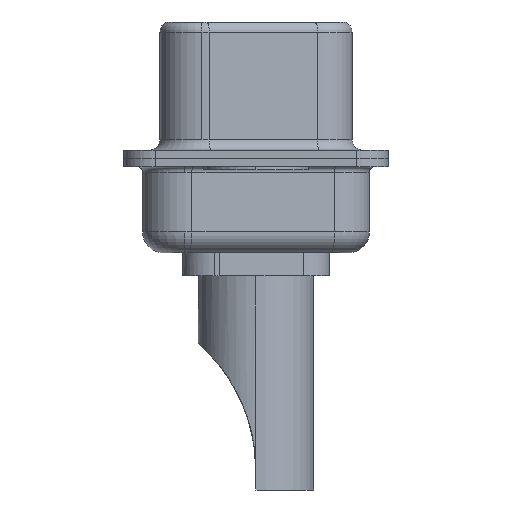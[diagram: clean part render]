
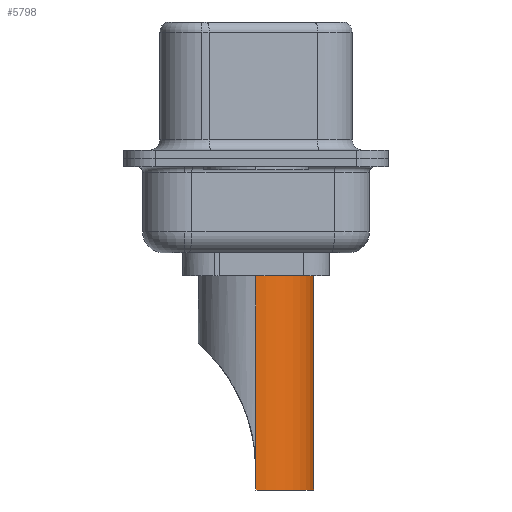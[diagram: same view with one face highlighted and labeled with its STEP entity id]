
A CAD part, left-side view. The second image highlights one B-rep face of the part: STEP entity #5798.
In plain terms, the highlighted cylindrical face has radius 2.75 mm (diameter 5.5 mm), a partial arc.
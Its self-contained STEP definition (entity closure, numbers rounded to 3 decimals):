
#401 = EDGE_CURVE ( 'NONE', #6301, #15592, #16591, .T. ) ;
#967 = CARTESIAN_POINT ( 'NONE',  ( 2.75, 0., -8.7 ) ) ;
#1114 = VECTOR ( 'NONE', #4449, 1000. ) ;
#1378 = ORIENTED_EDGE ( 'NONE', *, *, #10067, .F. ) ;
#1413 = CARTESIAN_POINT ( 'NONE',  ( 0., 0., -8.7 ) ) ;
#1638 = LINE ( 'NONE', #5240, #16275 ) ;
#2135 = EDGE_CURVE ( 'NONE', #3211, #16619, #16957, .T. ) ;
#2530 = EDGE_CURVE ( 'NONE', #3211, #7872, #1638, .T. ) ;
#2596 = DIRECTION ( 'NONE',  ( 0., 0., -1. ) ) ;
#3211 = VERTEX_POINT ( 'NONE', #11279 ) ;
#3229 = CARTESIAN_POINT ( 'NONE',  ( 2.75, 0., -8.7 ) ) ;
#3647 = DIRECTION ( 'NONE',  ( 0., 0., 1. ) ) ;
#3772 = DIRECTION ( 'NONE',  ( 1., 0., 0. ) ) ;
#3849 = VECTOR ( 'NONE', #13561, 1000. ) ;
#3994 = DIRECTION ( 'NONE',  ( 0., 0., 1. ) ) ;
#4449 = DIRECTION ( 'NONE',  ( 0., 0., -1. ) ) ;
#4693 = CIRCLE ( 'NONE', #11560, 2.75 ) ;
#5180 = LINE ( 'NONE', #3229, #1114 ) ;
#5205 = ORIENTED_EDGE ( 'NONE', *, *, #401, .T. ) ;
#5240 = CARTESIAN_POINT ( 'NONE',  ( -2.75, 0., -8.7 ) ) ;
#5243 = CARTESIAN_POINT ( 'NONE',  ( 2.75, 0., -7.764 ) ) ;
#5276 = DIRECTION ( 'NONE',  ( 0., 0., 1. ) ) ;
#5484 = DIRECTION ( 'NONE',  ( 1., 0., 0. ) ) ;
#5556 = CARTESIAN_POINT ( 'NONE',  ( 2.75, 0., 4.234 ) ) ;
#5577 = AXIS2_PLACEMENT_3D ( 'NONE', #1413, #3994, #5484 ) ;
#5798 = ADVANCED_FACE ( 'NONE', ( #11855 ), #17068, .T. ) ;
#6301 = VERTEX_POINT ( 'NONE', #5243 ) ;
#6537 = AXIS2_PLACEMENT_3D ( 'NONE', #12121, #5276, #3772 ) ;
#6841 = CARTESIAN_POINT ( 'NONE',  ( -2.75, 0., -8.7 ) ) ;
#7665 = EDGE_CURVE ( 'NONE', #6301, #13341, #5180, .T. ) ;
#7684 = DIRECTION ( 'NONE',  ( 1., 0., 0. ) ) ;
#7872 = VERTEX_POINT ( 'NONE', #6841 ) ;
#8949 = CARTESIAN_POINT ( 'NONE',  ( 0., 0., 1.5 ) ) ;
#9316 = ORIENTED_EDGE ( 'NONE', *, *, #16079, .T. ) ;
#9963 = DIRECTION ( 'NONE',  ( 0., 0., 1. ) ) ;
#10067 = EDGE_CURVE ( 'NONE', #16619, #15592, #4693, .T. ) ;
#10314 = ORIENTED_EDGE ( 'NONE', *, *, #7665, .F. ) ;
#10465 = EDGE_LOOP ( 'NONE', ( #16441, #12883, #9316, #10314, #5205, #1378 ) ) ;
#10871 = VECTOR ( 'NONE', #9963, 1000. ) ;
#11279 = CARTESIAN_POINT ( 'NONE',  ( -2.75, 0., -7.764 ) ) ;
#11560 = AXIS2_PLACEMENT_3D ( 'NONE', #8949, #3647, #7684 ) ;
#11855 = FACE_OUTER_BOUND ( 'NONE', #10465, .T. ) ;
#12052 = CARTESIAN_POINT ( 'NONE',  ( 2.75, 0., 1.5 ) ) ;
#12121 = CARTESIAN_POINT ( 'NONE',  ( 0., 0., 4.234 ) ) ;
#12450 = CIRCLE ( 'NONE', #5577, 2.75 ) ;
#12686 = CARTESIAN_POINT ( 'NONE',  ( -2.75, 0., 4.234 ) ) ;
#12883 = ORIENTED_EDGE ( 'NONE', *, *, #2530, .T. ) ;
#13341 = VERTEX_POINT ( 'NONE', #967 ) ;
#13561 = DIRECTION ( 'NONE',  ( 0., 0., 1. ) ) ;
#15592 = VERTEX_POINT ( 'NONE', #12052 ) ;
#16079 = EDGE_CURVE ( 'NONE', #7872, #13341, #12450, .T. ) ;
#16275 = VECTOR ( 'NONE', #2596, 1000. ) ;
#16441 = ORIENTED_EDGE ( 'NONE', *, *, #2135, .F. ) ;
#16591 = LINE ( 'NONE', #5556, #3849 ) ;
#16619 = VERTEX_POINT ( 'NONE', #17700 ) ;
#16957 = LINE ( 'NONE', #12686, #10871 ) ;
#17068 = CYLINDRICAL_SURFACE ( 'NONE', #6537, 2.75 ) ;
#17700 = CARTESIAN_POINT ( 'NONE',  ( -2.75, 0., 1.5 ) ) ;
